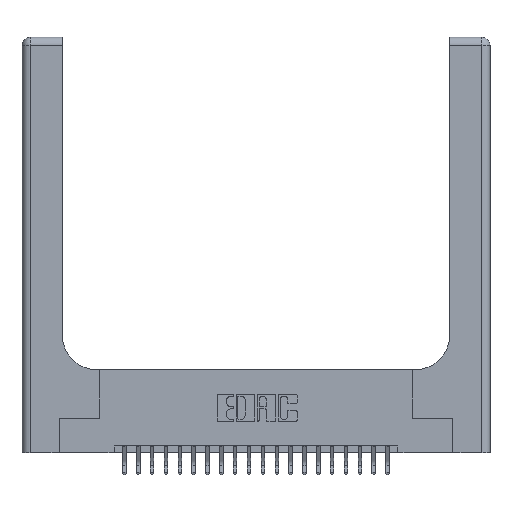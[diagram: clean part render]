
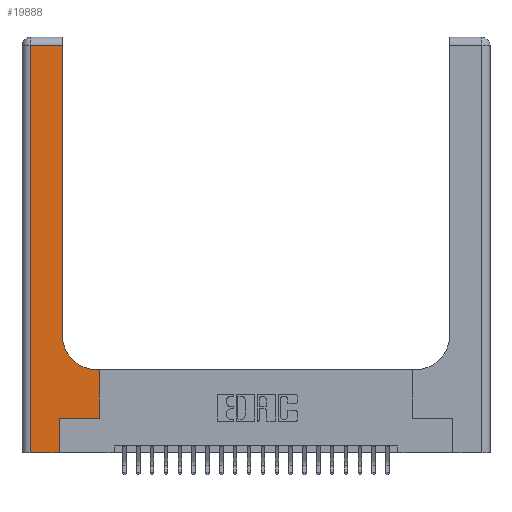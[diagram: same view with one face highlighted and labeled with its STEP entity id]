
A CAD part, top view. The second image highlights one B-rep face of the part: STEP entity #19888.
In plain terms, the highlighted planar face has unit normal (0, 0, 1).
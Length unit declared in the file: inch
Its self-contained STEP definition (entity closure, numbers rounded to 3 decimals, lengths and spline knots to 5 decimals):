
#95 = VECTOR ( 'NONE', #12414, 39.37008 ) ;
#1116 = CARTESIAN_POINT ( 'NONE',  ( 0.5415, 0.6, 0.37 ) ) ;
#1792 = VERTEX_POINT ( 'NONE', #17365 ) ;
#1849 = EDGE_CURVE ( 'NONE', #15688, #13360, #7643, .T. ) ;
#2158 = ORIENTED_EDGE ( 'NONE', *, *, #5327, .T. ) ;
#2501 = VECTOR ( 'NONE', #18654, 39.37008 ) ;
#2594 = CARTESIAN_POINT ( 'NONE',  ( 0.2915, 3., 0.37 ) ) ;
#2901 = CIRCLE ( 'NONE', #7164, 0.25 ) ;
#2906 = ORIENTED_EDGE ( 'NONE', *, *, #8484, .T. ) ;
#3569 = DIRECTION ( 'NONE',  ( -1., 0., 0. ) ) ;
#3789 = VERTEX_POINT ( 'NONE', #8622 ) ;
#3905 = ORIENTED_EDGE ( 'NONE', *, *, #1849, .T. ) ;
#4256 = VERTEX_POINT ( 'NONE', #1116 ) ;
#4803 = ORIENTED_EDGE ( 'NONE', *, *, #14999, .T. ) ;
#4996 = EDGE_LOOP ( 'NONE', ( #12789, #3905, #23802, #16854, #7235, #18872, #2158, #2906, #4803 ) ) ;
#5327 = EDGE_CURVE ( 'NONE', #11447, #1792, #17862, .T. ) ;
#6005 = EDGE_CURVE ( 'NONE', #21227, #20940, #18408, .T. ) ;
#6048 = DIRECTION ( 'NONE',  ( 0., 0., -1. ) ) ;
#6172 = CARTESIAN_POINT ( 'NONE',  ( 0.5585, 0.25, 0.37 ) ) ;
#6513 = EDGE_CURVE ( 'NONE', #3789, #15688, #8048, .T. ) ;
#6563 = VECTOR ( 'NONE', #11855, 39.37008 ) ;
#6925 = CARTESIAN_POINT ( 'NONE',  ( 0.269, 0., 0.37 ) ) ;
#7025 = DIRECTION ( 'NONE',  ( -1., 0., 0. ) ) ;
#7164 = AXIS2_PLACEMENT_3D ( 'NONE', #20663, #6048, #11460 ) ;
#7235 = ORIENTED_EDGE ( 'NONE', *, *, #6005, .T. ) ;
#7316 = DIRECTION ( 'NONE',  ( -1., 0., 0. ) ) ;
#7460 = VECTOR ( 'NONE', #15601, 39.37008 ) ;
#7536 = CARTESIAN_POINT ( 'NONE',  ( 0.269, 0., 0.37 ) ) ;
#7643 = LINE ( 'NONE', #19863, #11370 ) ;
#7757 = VECTOR ( 'NONE', #19398, 39.37008 ) ;
#8048 = LINE ( 'NONE', #2594, #7460 ) ;
#8484 = EDGE_CURVE ( 'NONE', #1792, #4256, #17500, .T. ) ;
#8622 = CARTESIAN_POINT ( 'NONE',  ( 0.2915, 0.85, 0.37 ) ) ;
#9736 = DIRECTION ( 'NONE',  ( 0., -1., 0. ) ) ;
#10701 = CARTESIAN_POINT ( 'NONE',  ( 0., 3., 0.37 ) ) ;
#10770 = AXIS2_PLACEMENT_3D ( 'NONE', #10701, #14725, #7316 ) ;
#11370 = VECTOR ( 'NONE', #7025, 39.37008 ) ;
#11447 = VERTEX_POINT ( 'NONE', #6172 ) ;
#11460 = DIRECTION ( 'NONE',  ( 1., 0., 0. ) ) ;
#11855 = DIRECTION ( 'NONE',  ( 0., 1., 0. ) ) ;
#12413 = LINE ( 'NONE', #18669, #2501 ) ;
#12414 = DIRECTION ( 'NONE',  ( 1., 0., 0. ) ) ;
#12789 = ORIENTED_EDGE ( 'NONE', *, *, #6513, .T. ) ;
#12918 = CARTESIAN_POINT ( 'NONE',  ( 0.2915, 0.6, 0.37 ) ) ;
#13360 = VERTEX_POINT ( 'NONE', #23959 ) ;
#14346 = LINE ( 'NONE', #20872, #15211 ) ;
#14725 = DIRECTION ( 'NONE',  ( 0., 0., -1. ) ) ;
#14774 = CARTESIAN_POINT ( 'NONE',  ( 0.06, 0., 0.37 ) ) ;
#14976 = VERTEX_POINT ( 'NONE', #14774 ) ;
#14999 = EDGE_CURVE ( 'NONE', #4256, #3789, #2901, .T. ) ;
#15211 = VECTOR ( 'NONE', #9736, 39.37008 ) ;
#15601 = DIRECTION ( 'NONE',  ( 0., 1., 0. ) ) ;
#15688 = VERTEX_POINT ( 'NONE', #16171 ) ;
#16171 = CARTESIAN_POINT ( 'NONE',  ( 0.2915, 2.94, 0.37 ) ) ;
#16854 = ORIENTED_EDGE ( 'NONE', *, *, #19109, .T. ) ;
#17365 = CARTESIAN_POINT ( 'NONE',  ( 0.5585, 0.6, 0.37 ) ) ;
#17500 = LINE ( 'NONE', #12918, #23340 ) ;
#17862 = LINE ( 'NONE', #20926, #7757 ) ;
#18036 = EDGE_CURVE ( 'NONE', #20940, #11447, #12413, .T. ) ;
#18408 = LINE ( 'NONE', #6925, #6563 ) ;
#18654 = DIRECTION ( 'NONE',  ( 1., 0., 0. ) ) ;
#18669 = CARTESIAN_POINT ( 'NONE',  ( 0.269, 0.25, 0.37 ) ) ;
#18872 = ORIENTED_EDGE ( 'NONE', *, *, #18036, .T. ) ;
#19109 = EDGE_CURVE ( 'NONE', #14976, #21227, #23391, .T. ) ;
#19398 = DIRECTION ( 'NONE',  ( 0., 1., 0. ) ) ;
#19661 = EDGE_CURVE ( 'NONE', #13360, #14976, #14346, .T. ) ;
#19711 = CARTESIAN_POINT ( 'NONE',  ( 0.269, 0.25, 0.37 ) ) ;
#19863 = CARTESIAN_POINT ( 'NONE',  ( 0., 2.94, 0.37 ) ) ;
#19888 = ADVANCED_FACE ( 'NONE', ( #23342 ), #23894, .F. ) ;
#20663 = CARTESIAN_POINT ( 'NONE',  ( 0.5415, 0.85, 0.37 ) ) ;
#20872 = CARTESIAN_POINT ( 'NONE',  ( 0.06, 3., 0.37 ) ) ;
#20926 = CARTESIAN_POINT ( 'NONE',  ( 0.5585, 0.25, 0.37 ) ) ;
#20940 = VERTEX_POINT ( 'NONE', #19711 ) ;
#21227 = VERTEX_POINT ( 'NONE', #7536 ) ;
#23340 = VECTOR ( 'NONE', #3569, 39.37008 ) ;
#23342 = FACE_OUTER_BOUND ( 'NONE', #4996, .T. ) ;
#23391 = LINE ( 'NONE', #23520, #95 ) ;
#23520 = CARTESIAN_POINT ( 'NONE',  ( 0., 0., 0.37 ) ) ;
#23802 = ORIENTED_EDGE ( 'NONE', *, *, #19661, .T. ) ;
#23894 = PLANE ( 'NONE',  #10770 ) ;
#23959 = CARTESIAN_POINT ( 'NONE',  ( 0.06, 2.94, 0.37 ) ) ;
